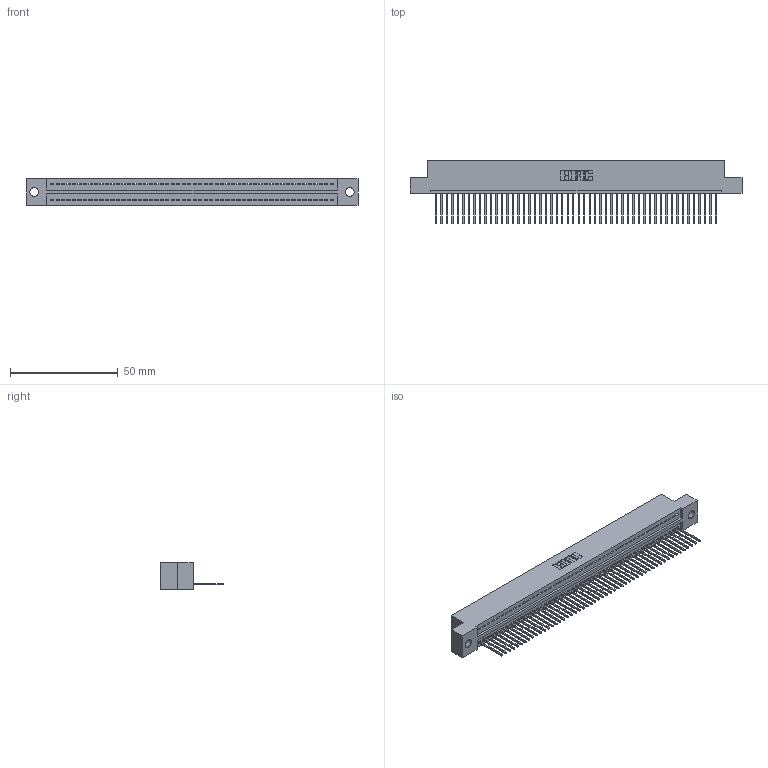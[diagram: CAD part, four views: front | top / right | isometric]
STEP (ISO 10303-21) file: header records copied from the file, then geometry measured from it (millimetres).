
FILE_DESCRIPTION (( 'STEP AP203' ), '1' );
FILE_NAME ('325-052-540-109.STEP', '2020-02-25T00:30:55', ( '' ), ( '' ), 'SwSTEP 2.0', 'SolidWorks 2016', '' );
FILE_SCHEMA (( 'CONFIG_CONTROL_DESIGN' ));
Length unit declared in the file: inch
Products named in the file (3): 325-052-540-109; 325 Part_.160 TH; 325-292-001_325-293-140
Assembly tree (53 placements, depth 2):
  325-052-540-109
    325 Part_.160 TH
    325-292-001_325-293-140  x52
Bounding box: 153.8 x 29.46 x 12.45 mm (x, y, z)
Volume: 19443 mm3; surface area: 21827.8 mm2
Topology: 53 solids, 53 shells, 3130 faces, 9463 edges, 6238 vertices
Faces by surface type: plane 2254, cylinder 876
Entity records: 30517 total; most frequent: CARTESIAN_POINT 5270, ORIENTED_EDGE 5258, DIRECTION 4425, EDGE_CURVE 2629, VECTOR 2501, LINE 2501, VERTEX_POINT 1750, AXIS2_PLACEMENT_3D 962
